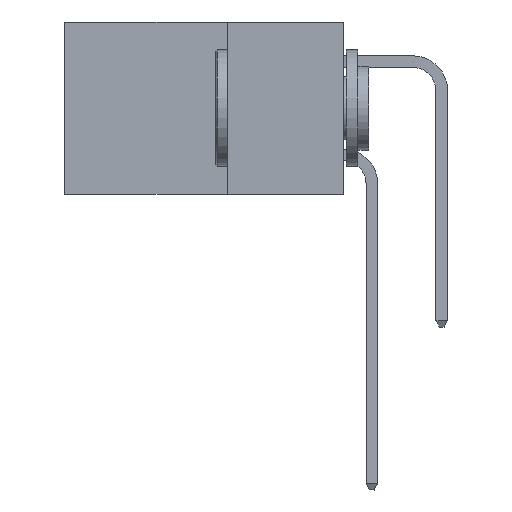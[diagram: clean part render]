
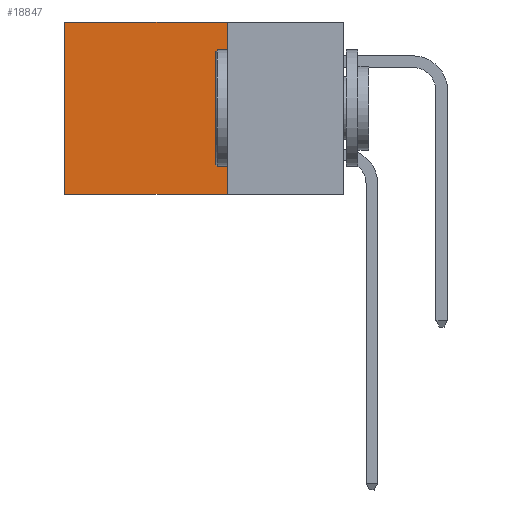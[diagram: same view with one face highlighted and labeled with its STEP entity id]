
A CAD part, left-side view. The second image highlights one B-rep face of the part: STEP entity #18847.
In plain terms, the highlighted planar face has unit normal (-1, 0, 0).
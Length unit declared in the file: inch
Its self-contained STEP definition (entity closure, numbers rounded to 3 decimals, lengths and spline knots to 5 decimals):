
#771 = ORIENTED_EDGE ( 'NONE', *, *, #17959, .F. ) ;
#1442 = DIRECTION ( 'NONE',  ( 0., 1., 0. ) ) ;
#4857 = VERTEX_POINT ( 'NONE', #11952 ) ;
#6062 = PLANE ( 'NONE',  #16135 ) ;
#6474 = VERTEX_POINT ( 'NONE', #13795 ) ;
#7174 = CARTESIAN_POINT ( 'NONE',  ( 0.298, 0.6, 0. ) ) ;
#7281 = CARTESIAN_POINT ( 'NONE',  ( 0.298, 0.25, -0.37 ) ) ;
#7989 = LINE ( 'NONE', #7174, #18202 ) ;
#8076 = DIRECTION ( 'NONE',  ( 0., 0., -1. ) ) ;
#8173 = CARTESIAN_POINT ( 'NONE',  ( 0.298, 0.25, 0. ) ) ;
#8478 = VECTOR ( 'NONE', #8076, 39.37008 ) ;
#8653 = VECTOR ( 'NONE', #23556, 39.37008 ) ;
#9309 = DIRECTION ( 'NONE',  ( 0., 0., -1. ) ) ;
#9824 = CARTESIAN_POINT ( 'NONE',  ( 0.298, 0.6, -0.37 ) ) ;
#9913 = ORIENTED_EDGE ( 'NONE', *, *, #25468, .T. ) ;
#10277 = DIRECTION ( 'NONE',  ( 0., 0., -1. ) ) ;
#11952 = CARTESIAN_POINT ( 'NONE',  ( 0.298, 0.25, 0. ) ) ;
#12296 = EDGE_LOOP ( 'NONE', ( #16433, #771, #22612, #9913 ) ) ;
#13010 = EDGE_CURVE ( 'NONE', #6474, #20618, #7989, .T. ) ;
#13795 = CARTESIAN_POINT ( 'NONE',  ( 0.298, 0.6, 0. ) ) ;
#13900 = VERTEX_POINT ( 'NONE', #16456 ) ;
#14559 = LINE ( 'NONE', #23956, #24616 ) ;
#16135 = AXIS2_PLACEMENT_3D ( 'NONE', #20370, #22395, #10277 ) ;
#16433 = ORIENTED_EDGE ( 'NONE', *, *, #13010, .T. ) ;
#16456 = CARTESIAN_POINT ( 'NONE',  ( 0.298, 0.25, -0.37 ) ) ;
#17959 = EDGE_CURVE ( 'NONE', #13900, #20618, #24808, .T. ) ;
#18202 = VECTOR ( 'NONE', #9309, 39.37008 ) ;
#18847 = ADVANCED_FACE ( 'NONE', ( #19436 ), #6062, .F. ) ;
#19305 = LINE ( 'NONE', #8173, #8478 ) ;
#19436 = FACE_OUTER_BOUND ( 'NONE', #12296, .T. ) ;
#20370 = CARTESIAN_POINT ( 'NONE',  ( 0.298, 0.25, 0. ) ) ;
#20618 = VERTEX_POINT ( 'NONE', #9824 ) ;
#22395 = DIRECTION ( 'NONE',  ( 1., 0., 0. ) ) ;
#22612 = ORIENTED_EDGE ( 'NONE', *, *, #25076, .F. ) ;
#23556 = DIRECTION ( 'NONE',  ( 0., 1., 0. ) ) ;
#23956 = CARTESIAN_POINT ( 'NONE',  ( 0.298, 0.25, 0. ) ) ;
#24616 = VECTOR ( 'NONE', #1442, 39.37008 ) ;
#24808 = LINE ( 'NONE', #7281, #8653 ) ;
#25076 = EDGE_CURVE ( 'NONE', #4857, #13900, #19305, .T. ) ;
#25468 = EDGE_CURVE ( 'NONE', #4857, #6474, #14559, .T. ) ;
